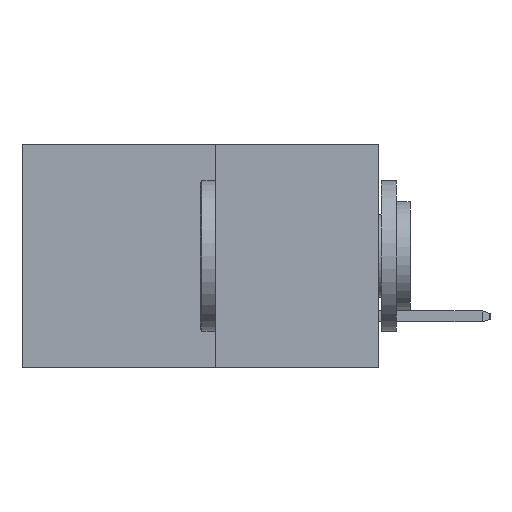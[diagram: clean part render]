
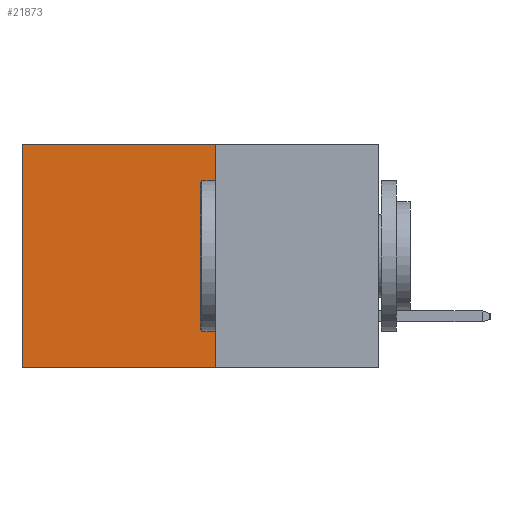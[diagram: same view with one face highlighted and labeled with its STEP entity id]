
A CAD part, left-side view. The second image highlights one B-rep face of the part: STEP entity #21873.
In plain terms, the highlighted planar face has unit normal (-1, 0, 0).
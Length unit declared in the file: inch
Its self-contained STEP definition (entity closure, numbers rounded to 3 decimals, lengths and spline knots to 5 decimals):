
#3712 = VECTOR ( 'NONE', #25561, 39.37008 ) ;
#3910 = VERTEX_POINT ( 'NONE', #21374 ) ;
#3958 = VERTEX_POINT ( 'NONE', #20213 ) ;
#4352 = CARTESIAN_POINT ( 'NONE',  ( 0.277, 0.27, 0. ) ) ;
#4463 = PLANE ( 'NONE',  #9575 ) ;
#4864 = VECTOR ( 'NONE', #22570, 39.37008 ) ;
#5664 = EDGE_CURVE ( 'NONE', #3910, #3958, #13886, .T. ) ;
#6627 = DIRECTION ( 'NONE',  ( 0., 0., -1. ) ) ;
#8417 = LINE ( 'NONE', #9659, #25093 ) ;
#8781 = VECTOR ( 'NONE', #13681, 39.37008 ) ;
#9202 = ORIENTED_EDGE ( 'NONE', *, *, #18797, .T. ) ;
#9575 = AXIS2_PLACEMENT_3D ( 'NONE', #23961, #19716, #6627 ) ;
#9659 = CARTESIAN_POINT ( 'NONE',  ( 0.277, 0.27, 0. ) ) ;
#10614 = LINE ( 'NONE', #13786, #4864 ) ;
#11834 = DIRECTION ( 'NONE',  ( 0., 1., 0. ) ) ;
#13681 = DIRECTION ( 'NONE',  ( 0., 1., 0. ) ) ;
#13786 = CARTESIAN_POINT ( 'NONE',  ( 0.277, 0.59, -0.37 ) ) ;
#13839 = CARTESIAN_POINT ( 'NONE',  ( 0.277, 0.27, -0.37 ) ) ;
#13886 = LINE ( 'NONE', #13839, #8781 ) ;
#14348 = CARTESIAN_POINT ( 'NONE',  ( 0.277, 0.59, 0. ) ) ;
#15148 = EDGE_CURVE ( 'NONE', #22258, #3958, #10614, .T. ) ;
#17195 = FACE_OUTER_BOUND ( 'NONE', #25226, .T. ) ;
#18037 = ORIENTED_EDGE ( 'NONE', *, *, #15148, .T. ) ;
#18797 = EDGE_CURVE ( 'NONE', #21046, #22258, #8417, .T. ) ;
#19716 = DIRECTION ( 'NONE',  ( 1., 0., 0. ) ) ;
#20213 = CARTESIAN_POINT ( 'NONE',  ( 0.277, 0.59, -0.37 ) ) ;
#21046 = VERTEX_POINT ( 'NONE', #4352 ) ;
#21343 = ORIENTED_EDGE ( 'NONE', *, *, #5664, .F. ) ;
#21374 = CARTESIAN_POINT ( 'NONE',  ( 0.277, 0.27, -0.37 ) ) ;
#21772 = LINE ( 'NONE', #23504, #3712 ) ;
#21873 = ADVANCED_FACE ( 'NONE', ( #17195 ), #4463, .F. ) ;
#22258 = VERTEX_POINT ( 'NONE', #14348 ) ;
#22570 = DIRECTION ( 'NONE',  ( 0., 0., -1. ) ) ;
#23504 = CARTESIAN_POINT ( 'NONE',  ( 0.277, 0.27, -0.37 ) ) ;
#23961 = CARTESIAN_POINT ( 'NONE',  ( 0.277, 0.27, -0.37 ) ) ;
#25093 = VECTOR ( 'NONE', #11834, 39.37008 ) ;
#25114 = ORIENTED_EDGE ( 'NONE', *, *, #26906, .F. ) ;
#25226 = EDGE_LOOP ( 'NONE', ( #18037, #21343, #25114, #9202 ) ) ;
#25561 = DIRECTION ( 'NONE',  ( 0., 0., -1. ) ) ;
#26906 = EDGE_CURVE ( 'NONE', #21046, #3910, #21772, .T. ) ;
